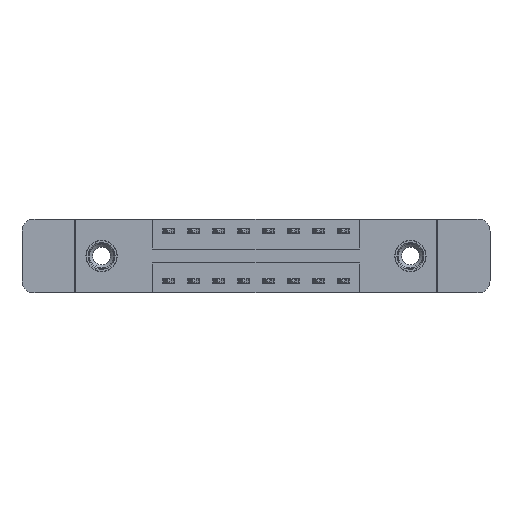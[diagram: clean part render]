
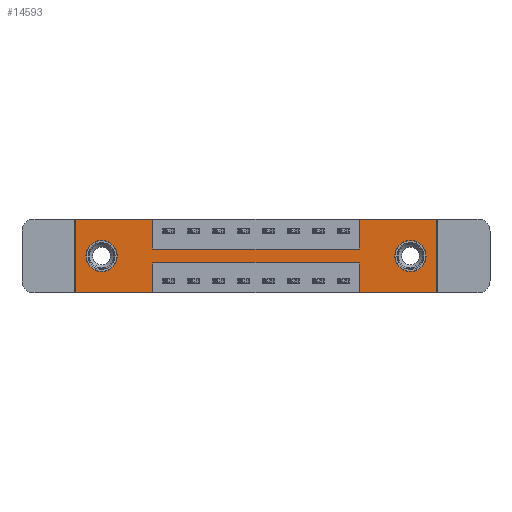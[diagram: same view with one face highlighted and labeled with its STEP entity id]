
A CAD part, front view. The second image highlights one B-rep face of the part: STEP entity #14593.
In plain terms, the highlighted planar face has unit normal (0, -1, 0).
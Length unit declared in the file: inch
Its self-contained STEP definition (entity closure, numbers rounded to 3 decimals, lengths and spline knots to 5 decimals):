
#12 = DIRECTION ( 'NONE',  ( 0., 0., -1. ) ) ;
#138 = VECTOR ( 'NONE', #14473, 39.37008 ) ;
#201 = DIRECTION ( 'NONE',  ( 0., 0., -1. ) ) ;
#259 = AXIS2_PLACEMENT_3D ( 'NONE', #11445, #11347, #11290 ) ;
#386 = CARTESIAN_POINT ( 'NONE',  ( 0.3875, 0., -0.15 ) ) ;
#417 = LINE ( 'NONE', #12608, #9753 ) ;
#475 = CARTESIAN_POINT ( 'NONE',  ( 1.6775, 0., -0.107 ) ) ;
#478 = CARTESIAN_POINT ( 'NONE',  ( 1.81, 0., 0. ) ) ;
#601 = CARTESIAN_POINT ( 'NONE',  ( 1.4225, 0., -0.15 ) ) ;
#713 = ORIENTED_EDGE ( 'NONE', *, *, #8457, .F. ) ;
#736 = EDGE_CURVE ( 'NONE', #4292, #1085, #6965, .T. ) ;
#909 = VECTOR ( 'NONE', #14625, 39.37008 ) ;
#989 = CARTESIAN_POINT ( 'NONE',  ( 0.3875, 0., -0.37 ) ) ;
#1043 = VERTEX_POINT ( 'NONE', #475 ) ;
#1085 = VERTEX_POINT ( 'NONE', #2801 ) ;
#1246 = VECTOR ( 'NONE', #7522, 39.37008 ) ;
#1448 = VERTEX_POINT ( 'NONE', #13714 ) ;
#1530 = EDGE_CURVE ( 'NONE', #1043, #9976, #14739, .T. ) ;
#1773 = VECTOR ( 'NONE', #14167, 39.37008 ) ;
#1783 = FACE_OUTER_BOUND ( 'NONE', #3359, .T. ) ;
#2330 = AXIS2_PLACEMENT_3D ( 'NONE', #12461, #11370, #4354 ) ;
#2416 = EDGE_CURVE ( 'NONE', #14655, #12869, #8564, .T. ) ;
#2435 = CIRCLE ( 'NONE', #2330, 0.078 ) ;
#2771 = DIRECTION ( 'NONE',  ( 0., 0., 1. ) ) ;
#2801 = CARTESIAN_POINT ( 'NONE',  ( 1.81, 0., -0.37 ) ) ;
#2863 = CARTESIAN_POINT ( 'NONE',  ( 1.4225, 0., 0. ) ) ;
#2957 = VERTEX_POINT ( 'NONE', #12111 ) ;
#2978 = CARTESIAN_POINT ( 'NONE',  ( 0.3875, 0., -0.22 ) ) ;
#3002 = EDGE_CURVE ( 'NONE', #5768, #11490, #13291, .T. ) ;
#3039 = CARTESIAN_POINT ( 'NONE',  ( 0.3875, 0., 0. ) ) ;
#3153 = CARTESIAN_POINT ( 'NONE',  ( 0., 0., 0. ) ) ;
#3188 = ORIENTED_EDGE ( 'NONE', *, *, #3246, .T. ) ;
#3246 = EDGE_CURVE ( 'NONE', #4029, #6269, #4320, .T. ) ;
#3298 = ORIENTED_EDGE ( 'NONE', *, *, #9040, .F. ) ;
#3309 = ORIENTED_EDGE ( 'NONE', *, *, #3002, .F. ) ;
#3359 = EDGE_LOOP ( 'NONE', ( #713, #9738, #12174, #8805, #5760, #12698, #3298, #3309, #9191, #13740, #5603, #8511 ) ) ;
#3373 = CARTESIAN_POINT ( 'NONE',  ( 0., 0., 0. ) ) ;
#3466 = VECTOR ( 'NONE', #5048, 39.37008 ) ;
#3539 = CARTESIAN_POINT ( 'NONE',  ( 0., 0., -0.37 ) ) ;
#3614 = CARTESIAN_POINT ( 'NONE',  ( 1.6775, 0., -0.185 ) ) ;
#3938 = CARTESIAN_POINT ( 'NONE',  ( 0.1325, 0., -0.107 ) ) ;
#4025 = CARTESIAN_POINT ( 'NONE',  ( 0.3875, 0., 0. ) ) ;
#4029 = VERTEX_POINT ( 'NONE', #6662 ) ;
#4068 = ORIENTED_EDGE ( 'NONE', *, *, #1530, .T. ) ;
#4081 = VECTOR ( 'NONE', #2771, 39.37008 ) ;
#4103 = DIRECTION ( 'NONE',  ( 1., 0., 0. ) ) ;
#4292 = VERTEX_POINT ( 'NONE', #478 ) ;
#4320 = CIRCLE ( 'NONE', #4983, 0.078 ) ;
#4354 = DIRECTION ( 'NONE',  ( 0., 0., 1. ) ) ;
#4363 = CARTESIAN_POINT ( 'NONE',  ( 1.81, 0., 0. ) ) ;
#4569 = DIRECTION ( 'NONE',  ( -1., 0., 0. ) ) ;
#4576 = CARTESIAN_POINT ( 'NONE',  ( 1.6775, 0., -0.263 ) ) ;
#4753 = DIRECTION ( 'NONE',  ( 0., 1., 0. ) ) ;
#4818 = FACE_BOUND ( 'NONE', #13415, .T. ) ;
#4983 = AXIS2_PLACEMENT_3D ( 'NONE', #11286, #5458, #13593 ) ;
#5010 = EDGE_CURVE ( 'NONE', #6269, #4029, #2435, .T. ) ;
#5048 = DIRECTION ( 'NONE',  ( 1., 0., 0. ) ) ;
#5169 = LINE ( 'NONE', #5977, #1773 ) ;
#5458 = DIRECTION ( 'NONE',  ( 0., 1., 0. ) ) ;
#5556 = FACE_BOUND ( 'NONE', #14379, .T. ) ;
#5580 = VECTOR ( 'NONE', #11332, 39.37008 ) ;
#5603 = ORIENTED_EDGE ( 'NONE', *, *, #14375, .F. ) ;
#5760 = ORIENTED_EDGE ( 'NONE', *, *, #736, .F. ) ;
#5768 = VERTEX_POINT ( 'NONE', #386 ) ;
#5803 = ORIENTED_EDGE ( 'NONE', *, *, #5010, .T. ) ;
#5966 = CARTESIAN_POINT ( 'NONE',  ( 0., 0., -0.37 ) ) ;
#5972 = VECTOR ( 'NONE', #201, 39.37008 ) ;
#5977 = CARTESIAN_POINT ( 'NONE',  ( 0., 0., -0.37 ) ) ;
#6012 = VERTEX_POINT ( 'NONE', #2863 ) ;
#6042 = EDGE_CURVE ( 'NONE', #10787, #10152, #8664, .T. ) ;
#6269 = VERTEX_POINT ( 'NONE', #3938 ) ;
#6662 = CARTESIAN_POINT ( 'NONE',  ( 0.1325, 0., -0.263 ) ) ;
#6689 = DIRECTION ( 'NONE',  ( 0., 0., -1. ) ) ;
#6965 = LINE ( 'NONE', #4363, #12811 ) ;
#7522 = DIRECTION ( 'NONE',  ( 0., 0., -1. ) ) ;
#7770 = LINE ( 'NONE', #14052, #5972 ) ;
#7809 = CARTESIAN_POINT ( 'NONE',  ( 0.3875, 0., -0.22 ) ) ;
#8457 = EDGE_CURVE ( 'NONE', #12078, #14655, #7770, .T. ) ;
#8511 = ORIENTED_EDGE ( 'NONE', *, *, #2416, .F. ) ;
#8564 = LINE ( 'NONE', #3539, #13135 ) ;
#8608 = ORIENTED_EDGE ( 'NONE', *, *, #9991, .T. ) ;
#8664 = LINE ( 'NONE', #3153, #5580 ) ;
#8805 = ORIENTED_EDGE ( 'NONE', *, *, #14854, .F. ) ;
#9015 = LINE ( 'NONE', #4025, #1246 ) ;
#9040 = EDGE_CURVE ( 'NONE', #11490, #6012, #13493, .T. ) ;
#9191 = ORIENTED_EDGE ( 'NONE', *, *, #13896, .F. ) ;
#9448 = CIRCLE ( 'NONE', #14760, 0.078 ) ;
#9704 = CARTESIAN_POINT ( 'NONE',  ( 1.4225, 0., -0.37 ) ) ;
#9737 = LINE ( 'NONE', #9704, #4081 ) ;
#9738 = ORIENTED_EDGE ( 'NONE', *, *, #13059, .F. ) ;
#9753 = VECTOR ( 'NONE', #4103, 39.37008 ) ;
#9976 = VERTEX_POINT ( 'NONE', #4576 ) ;
#9991 = EDGE_CURVE ( 'NONE', #9976, #1043, #9448, .T. ) ;
#10152 = VERTEX_POINT ( 'NONE', #3039 ) ;
#10407 = VECTOR ( 'NONE', #13033, 39.37008 ) ;
#10647 = CARTESIAN_POINT ( 'NONE',  ( 1.6775, 0., -0.185 ) ) ;
#10768 = EDGE_CURVE ( 'NONE', #6012, #4292, #417, .T. ) ;
#10787 = VERTEX_POINT ( 'NONE', #3373 ) ;
#10839 = CARTESIAN_POINT ( 'NONE',  ( 0., 0., 0. ) ) ;
#10889 = CARTESIAN_POINT ( 'NONE',  ( 0.3875, 0., -0.15 ) ) ;
#11245 = PLANE ( 'NONE',  #259 ) ;
#11286 = CARTESIAN_POINT ( 'NONE',  ( 0.1325, 0., -0.185 ) ) ;
#11290 = DIRECTION ( 'NONE',  ( 0., 0., -1. ) ) ;
#11332 = DIRECTION ( 'NONE',  ( 1., 0., 0. ) ) ;
#11347 = DIRECTION ( 'NONE',  ( 0., -1., 0. ) ) ;
#11370 = DIRECTION ( 'NONE',  ( 0., 1., 0. ) ) ;
#11445 = CARTESIAN_POINT ( 'NONE',  ( 0., 0., -0.37 ) ) ;
#11490 = VERTEX_POINT ( 'NONE', #601 ) ;
#11583 = LINE ( 'NONE', #10839, #138 ) ;
#12078 = VERTEX_POINT ( 'NONE', #2978 ) ;
#12111 = CARTESIAN_POINT ( 'NONE',  ( 1.4225, 0., -0.22 ) ) ;
#12174 = ORIENTED_EDGE ( 'NONE', *, *, #14428, .F. ) ;
#12179 = LINE ( 'NONE', #7809, #909 ) ;
#12461 = CARTESIAN_POINT ( 'NONE',  ( 0.1325, 0., -0.185 ) ) ;
#12608 = CARTESIAN_POINT ( 'NONE',  ( 0., 0., 0. ) ) ;
#12635 = AXIS2_PLACEMENT_3D ( 'NONE', #3614, #4753, #12 ) ;
#12698 = ORIENTED_EDGE ( 'NONE', *, *, #10768, .F. ) ;
#12811 = VECTOR ( 'NONE', #6689, 39.37008 ) ;
#12869 = VERTEX_POINT ( 'NONE', #5966 ) ;
#12978 = CARTESIAN_POINT ( 'NONE',  ( 1.4225, 0., 0. ) ) ;
#13033 = DIRECTION ( 'NONE',  ( 0., 0., 1. ) ) ;
#13059 = EDGE_CURVE ( 'NONE', #2957, #12078, #12179, .T. ) ;
#13135 = VECTOR ( 'NONE', #4569, 39.37008 ) ;
#13144 = DIRECTION ( 'NONE',  ( 0., 1., 0. ) ) ;
#13291 = LINE ( 'NONE', #10889, #3466 ) ;
#13415 = EDGE_LOOP ( 'NONE', ( #4068, #8608 ) ) ;
#13493 = LINE ( 'NONE', #12978, #10407 ) ;
#13593 = DIRECTION ( 'NONE',  ( 0., 0., 1. ) ) ;
#13714 = CARTESIAN_POINT ( 'NONE',  ( 1.4225, 0., -0.37 ) ) ;
#13740 = ORIENTED_EDGE ( 'NONE', *, *, #6042, .F. ) ;
#13896 = EDGE_CURVE ( 'NONE', #10152, #5768, #9015, .T. ) ;
#14052 = CARTESIAN_POINT ( 'NONE',  ( 0.3875, 0., -0.37 ) ) ;
#14167 = DIRECTION ( 'NONE',  ( -1., 0., 0. ) ) ;
#14305 = DIRECTION ( 'NONE',  ( 0., 0., -1. ) ) ;
#14375 = EDGE_CURVE ( 'NONE', #12869, #10787, #11583, .T. ) ;
#14379 = EDGE_LOOP ( 'NONE', ( #5803, #3188 ) ) ;
#14428 = EDGE_CURVE ( 'NONE', #1448, #2957, #9737, .T. ) ;
#14473 = DIRECTION ( 'NONE',  ( 0., 0., 1. ) ) ;
#14593 = ADVANCED_FACE ( 'NONE', ( #4818, #5556, #1783 ), #11245, .T. ) ;
#14625 = DIRECTION ( 'NONE',  ( -1., 0., 0. ) ) ;
#14655 = VERTEX_POINT ( 'NONE', #989 ) ;
#14739 = CIRCLE ( 'NONE', #12635, 0.078 ) ;
#14760 = AXIS2_PLACEMENT_3D ( 'NONE', #10647, #13144, #14305 ) ;
#14854 = EDGE_CURVE ( 'NONE', #1085, #1448, #5169, .T. ) ;
